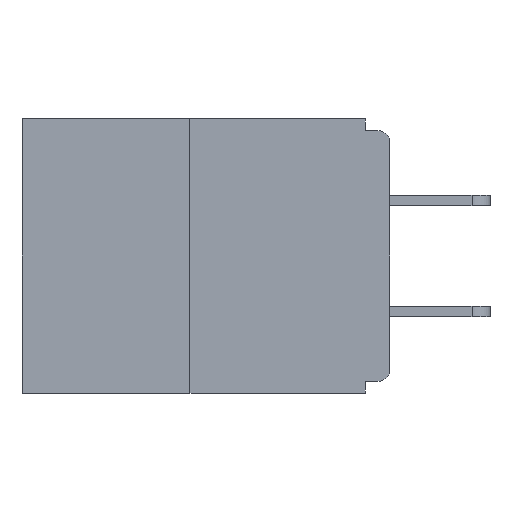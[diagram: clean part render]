
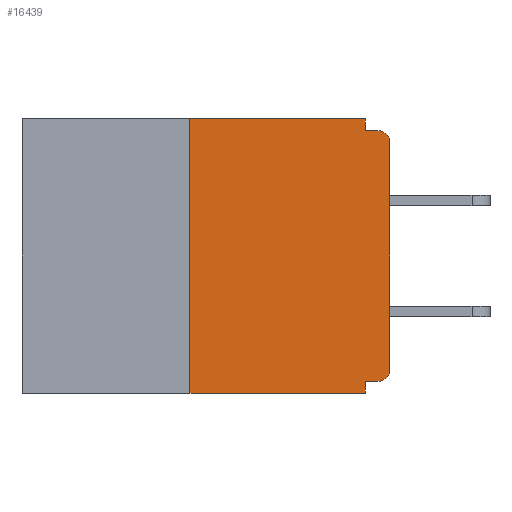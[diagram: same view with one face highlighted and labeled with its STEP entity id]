
A CAD part, left-side view. The second image highlights one B-rep face of the part: STEP entity #16439.
In plain terms, the highlighted planar face has unit normal (-1, 0, 0).
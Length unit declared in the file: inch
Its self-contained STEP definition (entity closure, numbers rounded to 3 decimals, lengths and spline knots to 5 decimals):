
#264 = EDGE_CURVE ( 'NONE', #8989, #8344, #5758, .T. ) ;
#500 = AXIS2_PLACEMENT_3D ( 'NONE', #4194, #5491, #8293 ) ;
#507 = CARTESIAN_POINT ( 'NONE',  ( 0., 0.25, -0.343 ) ) ;
#852 = DIRECTION ( 'NONE',  ( 0., -1., 0. ) ) ;
#910 = FACE_OUTER_BOUND ( 'NONE', #11817, .T. ) ;
#964 = ORIENTED_EDGE ( 'NONE', *, *, #15234, .F. ) ;
#1096 = EDGE_CURVE ( 'NONE', #6033, #12813, #4877, .T. ) ;
#1126 = CIRCLE ( 'NONE', #1977, 0.015 ) ;
#1388 = CARTESIAN_POINT ( 'NONE',  ( 0., 0.031, -0.343 ) ) ;
#1461 = DIRECTION ( 'NONE',  ( 0., 0., -1. ) ) ;
#1642 = CARTESIAN_POINT ( 'NONE',  ( 0., 0.25, 0. ) ) ;
#1977 = AXIS2_PLACEMENT_3D ( 'NONE', #17144, #3507, #17372 ) ;
#2148 = CIRCLE ( 'NONE', #15852, 0.015 ) ;
#2169 = LINE ( 'NONE', #11897, #10696 ) ;
#2501 = VERTEX_POINT ( 'NONE', #15808 ) ;
#2639 = CARTESIAN_POINT ( 'NONE',  ( 0., 0.031, 0. ) ) ;
#2998 = CARTESIAN_POINT ( 'NONE',  ( 0., 0.46, 0. ) ) ;
#3224 = ORIENTED_EDGE ( 'NONE', *, *, #264, .F. ) ;
#3280 = ORIENTED_EDGE ( 'NONE', *, *, #1096, .F. ) ;
#3397 = CARTESIAN_POINT ( 'NONE',  ( 0., 0., -0.015 ) ) ;
#3507 = DIRECTION ( 'NONE',  ( -1., 0., 0. ) ) ;
#4001 = EDGE_CURVE ( 'NONE', #5547, #7367, #2148, .T. ) ;
#4137 = PLANE ( 'NONE',  #500 ) ;
#4194 = CARTESIAN_POINT ( 'NONE',  ( 0., 0.46, 0. ) ) ;
#4877 = LINE ( 'NONE', #3397, #5513 ) ;
#4920 = LINE ( 'NONE', #1642, #17151 ) ;
#5362 = CARTESIAN_POINT ( 'NONE',  ( 0., 0.015, -0.313 ) ) ;
#5491 = DIRECTION ( 'NONE',  ( 1., 0., 0. ) ) ;
#5501 = VERTEX_POINT ( 'NONE', #14914 ) ;
#5513 = VECTOR ( 'NONE', #10210, 39.37008 ) ;
#5547 = VERTEX_POINT ( 'NONE', #12629 ) ;
#5758 = LINE ( 'NONE', #2998, #13911 ) ;
#5764 = LINE ( 'NONE', #2639, #12162 ) ;
#6033 = VERTEX_POINT ( 'NONE', #15400 ) ;
#6481 = EDGE_CURVE ( 'NONE', #5547, #5501, #6521, .T. ) ;
#6521 = LINE ( 'NONE', #16492, #14679 ) ;
#6609 = VECTOR ( 'NONE', #13754, 39.37008 ) ;
#7135 = CARTESIAN_POINT ( 'NONE',  ( 0., 0.031, 0. ) ) ;
#7367 = VERTEX_POINT ( 'NONE', #9308 ) ;
#7473 = LINE ( 'NONE', #16560, #6609 ) ;
#8286 = ORIENTED_EDGE ( 'NONE', *, *, #4001, .T. ) ;
#8293 = DIRECTION ( 'NONE',  ( 0., 0., -1. ) ) ;
#8344 = VERTEX_POINT ( 'NONE', #7135 ) ;
#8483 = VERTEX_POINT ( 'NONE', #507 ) ;
#8607 = DIRECTION ( 'NONE',  ( 0., 0., 1. ) ) ;
#8989 = VERTEX_POINT ( 'NONE', #13092 ) ;
#9308 = CARTESIAN_POINT ( 'NONE',  ( 0., 0., -0.313 ) ) ;
#9357 = LINE ( 'NONE', #1388, #12994 ) ;
#9451 = ORIENTED_EDGE ( 'NONE', *, *, #13602, .T. ) ;
#9665 = DIRECTION ( 'NONE',  ( 0., 1., 0. ) ) ;
#10210 = DIRECTION ( 'NONE',  ( 0., -1., 0. ) ) ;
#10418 = EDGE_CURVE ( 'NONE', #8483, #8989, #4920, .T. ) ;
#10581 = EDGE_CURVE ( 'NONE', #8483, #2501, #2169, .T. ) ;
#10696 = VECTOR ( 'NONE', #852, 39.37008 ) ;
#10817 = DIRECTION ( 'NONE',  ( -1., 0., 0. ) ) ;
#11020 = ORIENTED_EDGE ( 'NONE', *, *, #10581, .T. ) ;
#11051 = ORIENTED_EDGE ( 'NONE', *, *, #10418, .F. ) ;
#11434 = ORIENTED_EDGE ( 'NONE', *, *, #11615, .F. ) ;
#11615 = EDGE_CURVE ( 'NONE', #8344, #6033, #5764, .T. ) ;
#11817 = EDGE_LOOP ( 'NONE', ( #3224, #11051, #11020, #964, #16069, #8286, #9451, #12300, #3280, #11434 ) ) ;
#11897 = CARTESIAN_POINT ( 'NONE',  ( 0., 0.46, -0.343 ) ) ;
#12162 = VECTOR ( 'NONE', #17682, 39.37008 ) ;
#12300 = ORIENTED_EDGE ( 'NONE', *, *, #16117, .T. ) ;
#12629 = CARTESIAN_POINT ( 'NONE',  ( 0., 0.015, -0.328 ) ) ;
#12813 = VERTEX_POINT ( 'NONE', #13186 ) ;
#12994 = VECTOR ( 'NONE', #15133, 39.37008 ) ;
#13092 = CARTESIAN_POINT ( 'NONE',  ( 0., 0.25, 0. ) ) ;
#13186 = CARTESIAN_POINT ( 'NONE',  ( 0., 0.015, -0.015 ) ) ;
#13602 = EDGE_CURVE ( 'NONE', #7367, #14320, #7473, .T. ) ;
#13754 = DIRECTION ( 'NONE',  ( 0., 0., 1. ) ) ;
#13911 = VECTOR ( 'NONE', #16690, 39.37008 ) ;
#14320 = VERTEX_POINT ( 'NONE', #14397 ) ;
#14397 = CARTESIAN_POINT ( 'NONE',  ( 0., 0., -0.03 ) ) ;
#14679 = VECTOR ( 'NONE', #9665, 39.37008 ) ;
#14914 = CARTESIAN_POINT ( 'NONE',  ( 0., 0.031, -0.328 ) ) ;
#15133 = DIRECTION ( 'NONE',  ( 0., 0., -1. ) ) ;
#15234 = EDGE_CURVE ( 'NONE', #5501, #2501, #9357, .T. ) ;
#15400 = CARTESIAN_POINT ( 'NONE',  ( 0., 0.031, -0.015 ) ) ;
#15808 = CARTESIAN_POINT ( 'NONE',  ( 0., 0.031, -0.343 ) ) ;
#15852 = AXIS2_PLACEMENT_3D ( 'NONE', #5362, #10817, #1461 ) ;
#16069 = ORIENTED_EDGE ( 'NONE', *, *, #6481, .F. ) ;
#16117 = EDGE_CURVE ( 'NONE', #14320, #12813, #1126, .T. ) ;
#16439 = ADVANCED_FACE ( 'NONE', ( #910 ), #4137, .F. ) ;
#16492 = CARTESIAN_POINT ( 'NONE',  ( 0., 0., -0.328 ) ) ;
#16560 = CARTESIAN_POINT ( 'NONE',  ( 0., 0., 0. ) ) ;
#16690 = DIRECTION ( 'NONE',  ( 0., -1., 0. ) ) ;
#17144 = CARTESIAN_POINT ( 'NONE',  ( 0., 0.015, -0.03 ) ) ;
#17151 = VECTOR ( 'NONE', #8607, 39.37008 ) ;
#17372 = DIRECTION ( 'NONE',  ( 0., 0., -1. ) ) ;
#17682 = DIRECTION ( 'NONE',  ( 0., 0., -1. ) ) ;
